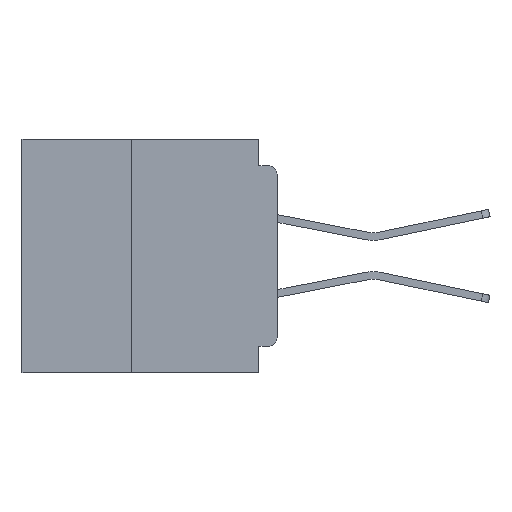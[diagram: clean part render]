
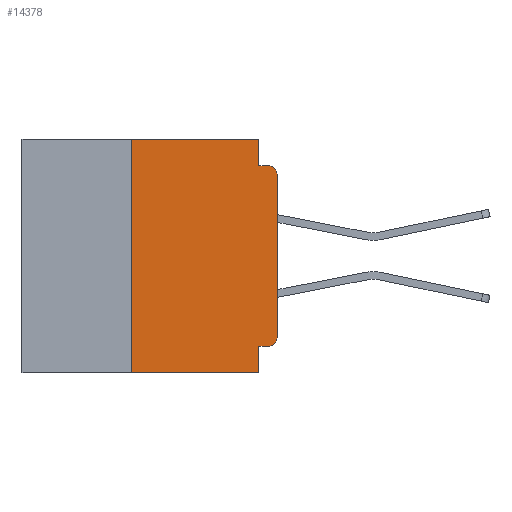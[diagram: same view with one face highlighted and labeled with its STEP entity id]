
A CAD part, left-side view. The second image highlights one B-rep face of the part: STEP entity #14378.
In plain terms, the highlighted planar face has unit normal (-1, 0, 0).
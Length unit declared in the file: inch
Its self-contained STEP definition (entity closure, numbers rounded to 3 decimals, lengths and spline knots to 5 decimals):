
#266 = CARTESIAN_POINT ( 'NONE',  ( 0., 0.031, -0.4 ) ) ;
#634 = DIRECTION ( 'NONE',  ( 0., 0., 1. ) ) ;
#920 = LINE ( 'NONE', #266, #28729 ) ;
#974 = VERTEX_POINT ( 'NONE', #28420 ) ;
#1061 = ORIENTED_EDGE ( 'NONE', *, *, #42339, .T. ) ;
#1823 = CARTESIAN_POINT ( 'NONE',  ( 0., 0.25, 0. ) ) ;
#1871 = VECTOR ( 'NONE', #20444, 39.37008 ) ;
#2328 = LINE ( 'NONE', #45791, #5187 ) ;
#3208 = CARTESIAN_POINT ( 'NONE',  ( 0., 0., -0.34 ) ) ;
#3231 = ORIENTED_EDGE ( 'NONE', *, *, #20962, .F. ) ;
#4362 = CARTESIAN_POINT ( 'NONE',  ( 0., 0., -0.06 ) ) ;
#4865 = LINE ( 'NONE', #46237, #13452 ) ;
#5080 = VECTOR ( 'NONE', #41111, 39.37008 ) ;
#5187 = VECTOR ( 'NONE', #17195, 39.37008 ) ;
#5213 = ORIENTED_EDGE ( 'NONE', *, *, #29452, .F. ) ;
#7583 = ORIENTED_EDGE ( 'NONE', *, *, #44549, .F. ) ;
#7936 = DIRECTION ( 'NONE',  ( 0., 0., -1. ) ) ;
#8924 = DIRECTION ( 'NONE',  ( -1., 0., 0. ) ) ;
#9283 = VERTEX_POINT ( 'NONE', #3208 ) ;
#10309 = VERTEX_POINT ( 'NONE', #24979 ) ;
#11438 = VERTEX_POINT ( 'NONE', #16851 ) ;
#11603 = CARTESIAN_POINT ( 'NONE',  ( 0., 0.015, -0.045 ) ) ;
#11612 = DIRECTION ( 'NONE',  ( 0., -1., 0. ) ) ;
#11742 = CARTESIAN_POINT ( 'NONE',  ( 0., 0.015, -0.355 ) ) ;
#11931 = EDGE_CURVE ( 'NONE', #28830, #9283, #27776, .T. ) ;
#12393 = DIRECTION ( 'NONE',  ( -1., 0., 0. ) ) ;
#13254 = FACE_OUTER_BOUND ( 'NONE', #39972, .T. ) ;
#13452 = VECTOR ( 'NONE', #24733, 39.37008 ) ;
#14114 = LINE ( 'NONE', #29537, #15250 ) ;
#14378 = ADVANCED_FACE ( 'NONE', ( #13254 ), #17466, .F. ) ;
#14430 = LINE ( 'NONE', #34700, #1871 ) ;
#14590 = ORIENTED_EDGE ( 'NONE', *, *, #11931, .T. ) ;
#15250 = VECTOR ( 'NONE', #7936, 39.37008 ) ;
#15952 = ORIENTED_EDGE ( 'NONE', *, *, #37989, .T. ) ;
#16851 = CARTESIAN_POINT ( 'NONE',  ( 0., 0.031, 0. ) ) ;
#17195 = DIRECTION ( 'NONE',  ( 0., 0., 1. ) ) ;
#17466 = PLANE ( 'NONE',  #40527 ) ;
#18368 = VERTEX_POINT ( 'NONE', #45564 ) ;
#18433 = DIRECTION ( 'NONE',  ( 0., 0., -1. ) ) ;
#19504 = VERTEX_POINT ( 'NONE', #35675 ) ;
#20444 = DIRECTION ( 'NONE',  ( 0., -1., 0. ) ) ;
#20962 = EDGE_CURVE ( 'NONE', #10309, #19504, #920, .T. ) ;
#21108 = DIRECTION ( 'NONE',  ( 1., 0., 0. ) ) ;
#23373 = VERTEX_POINT ( 'NONE', #4362 ) ;
#24496 = ORIENTED_EDGE ( 'NONE', *, *, #29890, .T. ) ;
#24733 = DIRECTION ( 'NONE',  ( 0., -1., 0. ) ) ;
#24979 = CARTESIAN_POINT ( 'NONE',  ( 0., 0.031, -0.355 ) ) ;
#26124 = AXIS2_PLACEMENT_3D ( 'NONE', #33924, #12393, #37548 ) ;
#27776 = CIRCLE ( 'NONE', #26124, 0.015 ) ;
#28001 = VECTOR ( 'NONE', #11612, 39.37008 ) ;
#28420 = CARTESIAN_POINT ( 'NONE',  ( 0., 0.031, -0.045 ) ) ;
#28729 = VECTOR ( 'NONE', #18433, 39.37008 ) ;
#28766 = EDGE_CURVE ( 'NONE', #11438, #974, #14114, .T. ) ;
#28830 = VERTEX_POINT ( 'NONE', #11742 ) ;
#29452 = EDGE_CURVE ( 'NONE', #18368, #45986, #43192, .T. ) ;
#29537 = CARTESIAN_POINT ( 'NONE',  ( 0., 0.031, 0. ) ) ;
#29890 = EDGE_CURVE ( 'NONE', #18368, #19504, #4865, .T. ) ;
#30012 = AXIS2_PLACEMENT_3D ( 'NONE', #30490, #8924, #34076 ) ;
#30490 = CARTESIAN_POINT ( 'NONE',  ( 0., 0.015, -0.06 ) ) ;
#30670 = ORIENTED_EDGE ( 'NONE', *, *, #37782, .F. ) ;
#31175 = EDGE_CURVE ( 'NONE', #974, #32661, #14430, .T. ) ;
#32661 = VERTEX_POINT ( 'NONE', #11603 ) ;
#32992 = CARTESIAN_POINT ( 'NONE',  ( 0., 0.437, 0. ) ) ;
#33008 = CIRCLE ( 'NONE', #30012, 0.015 ) ;
#33896 = LINE ( 'NONE', #37573, #5080 ) ;
#33924 = CARTESIAN_POINT ( 'NONE',  ( 0., 0.015, -0.34 ) ) ;
#34076 = DIRECTION ( 'NONE',  ( 0., 0., -1. ) ) ;
#34700 = CARTESIAN_POINT ( 'NONE',  ( 0., 0., -0.045 ) ) ;
#35675 = CARTESIAN_POINT ( 'NONE',  ( 0., 0.031, -0.4 ) ) ;
#36689 = CARTESIAN_POINT ( 'NONE',  ( 0., 0.25, -0.4 ) ) ;
#37372 = ORIENTED_EDGE ( 'NONE', *, *, #28766, .F. ) ;
#37528 = LINE ( 'NONE', #32992, #28001 ) ;
#37548 = DIRECTION ( 'NONE',  ( 0., 0., -1. ) ) ;
#37573 = CARTESIAN_POINT ( 'NONE',  ( 0., 0., -0.355 ) ) ;
#37782 = EDGE_CURVE ( 'NONE', #45986, #11438, #37528, .T. ) ;
#37989 = EDGE_CURVE ( 'NONE', #23373, #32661, #33008, .T. ) ;
#38430 = ORIENTED_EDGE ( 'NONE', *, *, #31175, .F. ) ;
#39972 = EDGE_LOOP ( 'NONE', ( #1061, #15952, #38430, #37372, #30670, #5213, #24496, #3231, #7583, #14590 ) ) ;
#40527 = AXIS2_PLACEMENT_3D ( 'NONE', #42501, #21108, #46057 ) ;
#41111 = DIRECTION ( 'NONE',  ( 0., 1., 0. ) ) ;
#42084 = VECTOR ( 'NONE', #634, 39.37008 ) ;
#42339 = EDGE_CURVE ( 'NONE', #9283, #23373, #2328, .T. ) ;
#42501 = CARTESIAN_POINT ( 'NONE',  ( 0., 0.437, 0. ) ) ;
#43192 = LINE ( 'NONE', #36689, #42084 ) ;
#44549 = EDGE_CURVE ( 'NONE', #28830, #10309, #33896, .T. ) ;
#45564 = CARTESIAN_POINT ( 'NONE',  ( 0., 0.25, -0.4 ) ) ;
#45791 = CARTESIAN_POINT ( 'NONE',  ( 0., 0., 0. ) ) ;
#45986 = VERTEX_POINT ( 'NONE', #1823 ) ;
#46057 = DIRECTION ( 'NONE',  ( 0., 0., -1. ) ) ;
#46237 = CARTESIAN_POINT ( 'NONE',  ( 0., 0.437, -0.4 ) ) ;
